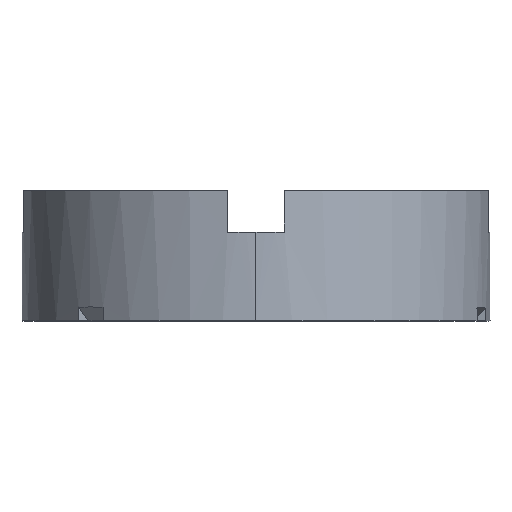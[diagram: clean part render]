
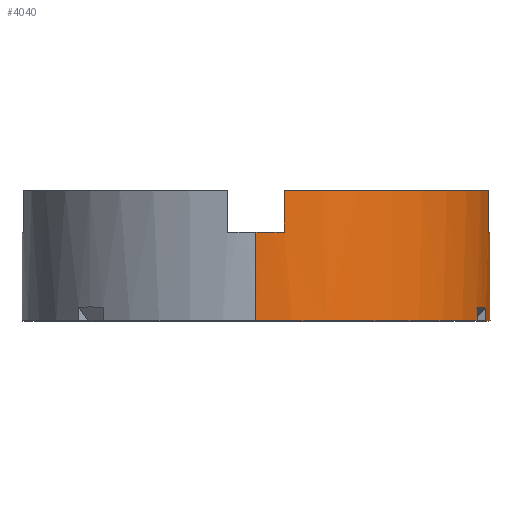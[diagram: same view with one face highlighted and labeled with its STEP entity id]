
A CAD part, top view. The second image highlights one B-rep face of the part: STEP entity #4040.
In plain terms, the highlighted cylindrical face has radius 17.209 mm (diameter 34.417 mm), a partial arc.
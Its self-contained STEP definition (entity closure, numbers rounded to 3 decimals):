
#107 = ORIENTED_EDGE ( 'NONE', *, *, #437, .T. ) ;
#111 = AXIS2_PLACEMENT_3D ( 'NONE', #4253, #3938, #3336 ) ;
#128 = CARTESIAN_POINT ( 'NONE',  ( 16.906, 0., 3.215 ) ) ;
#132 = AXIS2_PLACEMENT_3D ( 'NONE', #319, #4246, #3917 ) ;
#145 = VERTEX_POINT ( 'NONE', #3815 ) ;
#160 = AXIS2_PLACEMENT_3D ( 'NONE', #2483, #1819, #1105 ) ;
#173 = AXIS2_PLACEMENT_3D ( 'NONE', #3788, #3770, #3472 ) ;
#190 = AXIS2_PLACEMENT_3D ( 'NONE', #1860, #1522, #2311 ) ;
#206 = CARTESIAN_POINT ( 'NONE',  ( 0., 0., -17.208 ) ) ;
#232 = AXIS2_PLACEMENT_3D ( 'NONE', #1627, #2927, #2292 ) ;
#240 = DIRECTION ( 'NONE',  ( 0., 1., 0. ) ) ;
#242 = LINE ( 'NONE', #3937, #2090 ) ;
#274 = AXIS2_PLACEMENT_3D ( 'NONE', #2400, #2084, #2050 ) ;
#277 = DIRECTION ( 'NONE',  ( 0., -1., 0. ) ) ;
#293 = CARTESIAN_POINT ( 'NONE',  ( 16.906, 0.969, 3.215 ) ) ;
#319 = CARTESIAN_POINT ( 'NONE',  ( 0., 9.55, 0. ) ) ;
#320 = LINE ( 'NONE', #957, #556 ) ;
#346 = EDGE_CURVE ( 'NONE', #1330, #1467, #438, .T. ) ;
#358 = EDGE_CURVE ( 'NONE', #1058, #1961, #320, .T. ) ;
#362 = EDGE_CURVE ( 'NONE', #1498, #145, #1343, .T. ) ;
#368 = EDGE_CURVE ( 'NONE', #1330, #400, #3769, .T. ) ;
#375 = EDGE_CURVE ( 'NONE', #145, #3098, #1628, .T. ) ;
#382 = EDGE_CURVE ( 'NONE', #1991, #1040, #3672, .T. ) ;
#395 = VECTOR ( 'NONE', #277, 1000. ) ;
#397 = EDGE_CURVE ( 'NONE', #771, #400, #2899, .T. ) ;
#400 = VERTEX_POINT ( 'NONE', #3416 ) ;
#409 = EDGE_CURVE ( 'NONE', #800, #1991, #1946, .T. ) ;
#427 = EDGE_CURVE ( 'NONE', #1040, #1498, #3580, .T. ) ;
#434 = EDGE_CURVE ( 'NONE', #1285, #1058, #2715, .T. ) ;
#437 = EDGE_CURVE ( 'NONE', #1467, #1285, #4322, .T. ) ;
#438 = CIRCLE ( 'NONE', #274, 17.208 ) ;
#445 = EDGE_CURVE ( 'NONE', #1961, #3141, #1426, .T. ) ;
#458 = EDGE_CURVE ( 'NONE', #3141, #3449, #3829, .T. ) ;
#470 = ORIENTED_EDGE ( 'NONE', *, *, #375, .T. ) ;
#471 = EDGE_CURVE ( 'NONE', #3449, #4221, #3049, .T. ) ;
#477 = EDGE_CURVE ( 'NONE', #4221, #800, #2952, .T. ) ;
#556 = VECTOR ( 'NONE', #593, 1000. ) ;
#593 = DIRECTION ( 'NONE',  ( 0., -1., 0. ) ) ;
#601 = CARTESIAN_POINT ( 'NONE',  ( 2.096, 9.55, -17.08 ) ) ;
#674 = AXIS2_PLACEMENT_3D ( 'NONE', #699, #682, #2790 ) ;
#682 = DIRECTION ( 'NONE',  ( 0., -1., 0. ) ) ;
#699 = CARTESIAN_POINT ( 'NONE',  ( 0., 0., 0. ) ) ;
#771 = VERTEX_POINT ( 'NONE', #128 ) ;
#775 = FACE_OUTER_BOUND ( 'NONE', #3735, .T. ) ;
#787 = ORIENTED_EDGE ( 'NONE', *, *, #445, .T. ) ;
#800 = VERTEX_POINT ( 'NONE', #3812 ) ;
#957 = CARTESIAN_POINT ( 'NONE',  ( 17.08, 0., -2.096 ) ) ;
#994 = CARTESIAN_POINT ( 'NONE',  ( 16.248, 0.969, 5.668 ) ) ;
#1007 = ORIENTED_EDGE ( 'NONE', *, *, #346, .T. ) ;
#1009 = CARTESIAN_POINT ( 'NONE',  ( 17.08, 0., 2.095 ) ) ;
#1030 = CARTESIAN_POINT ( 'NONE',  ( 2.096, 0., 17.08 ) ) ;
#1040 = VERTEX_POINT ( 'NONE', #3521 ) ;
#1052 = CARTESIAN_POINT ( 'NONE',  ( 0., 6.502, -17.208 ) ) ;
#1058 = VERTEX_POINT ( 'NONE', #1717 ) ;
#1073 = DIRECTION ( 'NONE',  ( 0., 1., 0. ) ) ;
#1105 = DIRECTION ( 'NONE',  ( 0., 0., -1. ) ) ;
#1127 = DIRECTION ( 'NONE',  ( 0., -1., 0. ) ) ;
#1222 = VECTOR ( 'NONE', #1127, 1000. ) ;
#1235 = CARTESIAN_POINT ( 'NONE',  ( 2.096, 0., -17.08 ) ) ;
#1285 = VERTEX_POINT ( 'NONE', #601 ) ;
#1330 = VERTEX_POINT ( 'NONE', #1052 ) ;
#1343 = LINE ( 'NONE', #2701, #2988 ) ;
#1355 = CARTESIAN_POINT ( 'NONE',  ( 16.528, 1.032, 4.868 ) ) ;
#1377 = ORIENTED_EDGE ( 'NONE', *, *, #368, .F. ) ;
#1426 = CIRCLE ( 'NONE', #160, 17.208 ) ;
#1462 = CARTESIAN_POINT ( 'NONE',  ( 17.08, 6.502, 2.095 ) ) ;
#1467 = VERTEX_POINT ( 'NONE', #2420 ) ;
#1497 = ORIENTED_EDGE ( 'NONE', *, *, #382, .T. ) ;
#1498 = VERTEX_POINT ( 'NONE', #3065 ) ;
#1522 = DIRECTION ( 'NONE',  ( 0., 1., 0. ) ) ;
#1627 = CARTESIAN_POINT ( 'NONE',  ( 0., 0., 0. ) ) ;
#1628 =( BOUNDED_CURVE ( )  B_SPLINE_CURVE ( 3, ( #994, #1355, #4365, #2237 ),
 .UNSPECIFIED., .F., .F. ) 
 B_SPLINE_CURVE_WITH_KNOTS ( ( 4, 4 ),
 ( 3.068, 3.215 ),
 .UNSPECIFIED. ) 
 CURVE ( )  GEOMETRIC_REPRESENTATION_ITEM ( )  RATIONAL_B_SPLINE_CURVE ( ( 1., 0.998, 0.998, 1. ) ) 
 REPRESENTATION_ITEM ( '' )  );
#1646 = DIRECTION ( 'NONE',  ( 0., 1., 0. ) ) ;
#1656 = ORIENTED_EDGE ( 'NONE', *, *, #477, .T. ) ;
#1717 = CARTESIAN_POINT ( 'NONE',  ( 17.08, 9.55, -2.096 ) ) ;
#1819 = DIRECTION ( 'NONE',  ( 0., -1., 0. ) ) ;
#1828 = CARTESIAN_POINT ( 'NONE',  ( 0., 6.502, 17.208 ) ) ;
#1854 = CARTESIAN_POINT ( 'NONE',  ( 2.096, 9.55, 17.08 ) ) ;
#1860 = CARTESIAN_POINT ( 'NONE',  ( 0., 0., 0. ) ) ;
#1946 = CIRCLE ( 'NONE', #173, 17.208 ) ;
#1961 = VERTEX_POINT ( 'NONE', #2143 ) ;
#1991 = VERTEX_POINT ( 'NONE', #1828 ) ;
#2050 = DIRECTION ( 'NONE',  ( 0., 0., -1. ) ) ;
#2084 = DIRECTION ( 'NONE',  ( 0., -1., 0. ) ) ;
#2090 = VECTOR ( 'NONE', #4269, 1000. ) ;
#2143 = CARTESIAN_POINT ( 'NONE',  ( 17.08, 6.502, -2.096 ) ) ;
#2153 = VECTOR ( 'NONE', #2848, 1000. ) ;
#2237 = CARTESIAN_POINT ( 'NONE',  ( 16.906, 0.969, 3.215 ) ) ;
#2292 = DIRECTION ( 'NONE',  ( 0., 0., -1. ) ) ;
#2304 = ORIENTED_EDGE ( 'NONE', *, *, #362, .T. ) ;
#2311 = DIRECTION ( 'NONE',  ( 0., 0., -1. ) ) ;
#2348 = VECTOR ( 'NONE', #1073, 1000. ) ;
#2400 = CARTESIAN_POINT ( 'NONE',  ( 0., 6.502, 0. ) ) ;
#2420 = CARTESIAN_POINT ( 'NONE',  ( 2.096, 6.502, -17.08 ) ) ;
#2483 = CARTESIAN_POINT ( 'NONE',  ( 0., 6.502, 0. ) ) ;
#2499 = EDGE_CURVE ( 'NONE', #3098, #771, #242, .T. ) ;
#2572 = CYLINDRICAL_SURFACE ( 'NONE', #674, 17.208 ) ;
#2701 = CARTESIAN_POINT ( 'NONE',  ( 16.248, 0., 5.668 ) ) ;
#2715 = CIRCLE ( 'NONE', #132, 17.208 ) ;
#2790 = DIRECTION ( 'NONE',  ( 0., 0., -1. ) ) ;
#2848 = DIRECTION ( 'NONE',  ( 0., -1., 0. ) ) ;
#2899 = CIRCLE ( 'NONE', #190, 17.208 ) ;
#2916 = ORIENTED_EDGE ( 'NONE', *, *, #2499, .T. ) ;
#2927 = DIRECTION ( 'NONE',  ( 0., 1., 0. ) ) ;
#2952 = LINE ( 'NONE', #1030, #395 ) ;
#2988 = VECTOR ( 'NONE', #240, 1000. ) ;
#3005 = ORIENTED_EDGE ( 'NONE', *, *, #427, .T. ) ;
#3015 = ORIENTED_EDGE ( 'NONE', *, *, #434, .T. ) ;
#3049 = CIRCLE ( 'NONE', #111, 17.208 ) ;
#3065 = CARTESIAN_POINT ( 'NONE',  ( 16.248, 0., 5.668 ) ) ;
#3098 = VERTEX_POINT ( 'NONE', #293 ) ;
#3111 = CARTESIAN_POINT ( 'NONE',  ( 0., 0., 17.208 ) ) ;
#3141 = VERTEX_POINT ( 'NONE', #1462 ) ;
#3195 = ORIENTED_EDGE ( 'NONE', *, *, #458, .T. ) ;
#3332 = ORIENTED_EDGE ( 'NONE', *, *, #471, .T. ) ;
#3336 = DIRECTION ( 'NONE',  ( 0., 0., -1. ) ) ;
#3413 = ORIENTED_EDGE ( 'NONE', *, *, #358, .T. ) ;
#3416 = CARTESIAN_POINT ( 'NONE',  ( 0., 0., -17.208 ) ) ;
#3449 = VERTEX_POINT ( 'NONE', #3654 ) ;
#3472 = DIRECTION ( 'NONE',  ( 0., 0., -1. ) ) ;
#3521 = CARTESIAN_POINT ( 'NONE',  ( 0., 0., 17.208 ) ) ;
#3580 = CIRCLE ( 'NONE', #232, 17.208 ) ;
#3654 = CARTESIAN_POINT ( 'NONE',  ( 17.08, 9.55, 2.095 ) ) ;
#3672 = LINE ( 'NONE', #3111, #2153 ) ;
#3694 = ORIENTED_EDGE ( 'NONE', *, *, #397, .T. ) ;
#3735 = EDGE_LOOP ( 'NONE', ( #3985, #1497, #3005, #2304, #470, #2916, #3694, #1377, #1007, #107, #3015, #3413, #787, #3195, #3332, #1656 ) ) ;
#3769 = LINE ( 'NONE', #206, #1222 ) ;
#3770 = DIRECTION ( 'NONE',  ( 0., -1., 0. ) ) ;
#3788 = CARTESIAN_POINT ( 'NONE',  ( 0., 6.502, 0. ) ) ;
#3812 = CARTESIAN_POINT ( 'NONE',  ( 2.096, 6.502, 17.08 ) ) ;
#3815 = CARTESIAN_POINT ( 'NONE',  ( 16.248, 0.969, 5.668 ) ) ;
#3829 = LINE ( 'NONE', #1009, #2348 ) ;
#3906 = VECTOR ( 'NONE', #1646, 1000. ) ;
#3917 = DIRECTION ( 'NONE',  ( 0., 0., -1. ) ) ;
#3937 = CARTESIAN_POINT ( 'NONE',  ( 16.906, 0., 3.215 ) ) ;
#3938 = DIRECTION ( 'NONE',  ( 0., -1., 0. ) ) ;
#3985 = ORIENTED_EDGE ( 'NONE', *, *, #409, .T. ) ;
#4040 = ADVANCED_FACE ( 'NONE', ( #775 ), #2572, .T. ) ;
#4221 = VERTEX_POINT ( 'NONE', #1854 ) ;
#4246 = DIRECTION ( 'NONE',  ( 0., -1., 0. ) ) ;
#4253 = CARTESIAN_POINT ( 'NONE',  ( 0., 9.55, 0. ) ) ;
#4269 = DIRECTION ( 'NONE',  ( 0., -1., 0. ) ) ;
#4322 = LINE ( 'NONE', #1235, #3906 ) ;
#4365 = CARTESIAN_POINT ( 'NONE',  ( 16.747, 1.032, 4.048 ) ) ;
